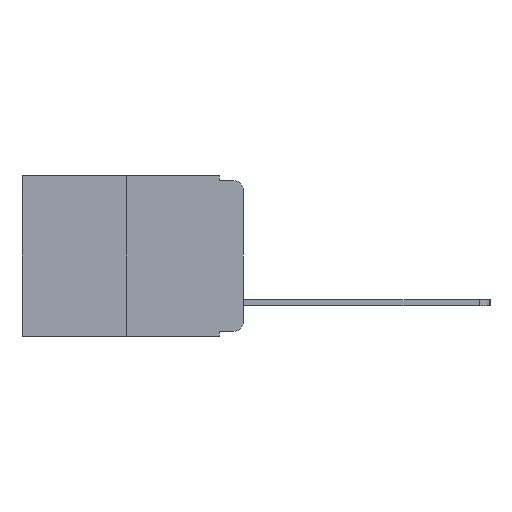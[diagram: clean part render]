
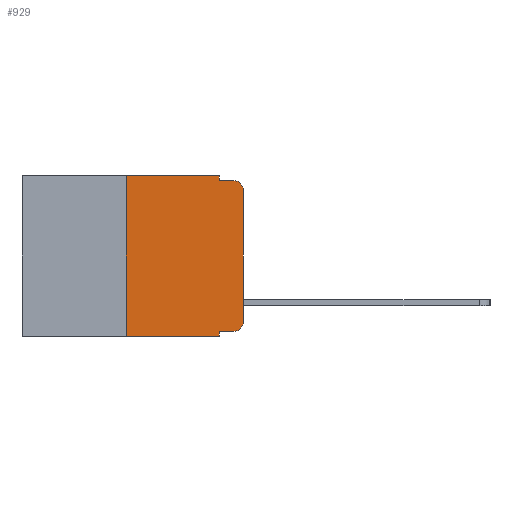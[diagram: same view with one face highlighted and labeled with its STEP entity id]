
A CAD part, left-side view. The second image highlights one B-rep face of the part: STEP entity #929.
In plain terms, the highlighted planar face has unit normal (-1, 0, 0).
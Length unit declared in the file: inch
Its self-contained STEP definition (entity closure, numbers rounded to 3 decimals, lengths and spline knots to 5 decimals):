
#144 = CARTESIAN_POINT ( 'NONE',  ( 0., 0.051, 0. ) ) ;
#150 = VECTOR ( 'NONE', #14400, 39.37008 ) ;
#474 = EDGE_CURVE ( 'NONE', #17470, #11154, #4488, .T. ) ;
#929 = ADVANCED_FACE ( 'NONE', ( #9199 ), #10557, .F. ) ;
#1122 = VERTEX_POINT ( 'NONE', #2299 ) ;
#1246 = CIRCLE ( 'NONE', #18736, 0.02 ) ;
#1361 = DIRECTION ( 'NONE',  ( -1., 0., 0. ) ) ;
#1369 = DIRECTION ( 'NONE',  ( 0., -1., 0. ) ) ;
#1697 = CARTESIAN_POINT ( 'NONE',  ( 0., 0.02, -0.03 ) ) ;
#2299 = CARTESIAN_POINT ( 'NONE',  ( 0., 0.051, -0.333 ) ) ;
#2404 = LINE ( 'NONE', #7173, #10400 ) ;
#2425 = DIRECTION ( 'NONE',  ( 0., 0., -1. ) ) ;
#2834 = VECTOR ( 'NONE', #5025, 39.37008 ) ;
#2888 = ORIENTED_EDGE ( 'NONE', *, *, #14302, .F. ) ;
#3519 = VECTOR ( 'NONE', #6937, 39.37008 ) ;
#3643 = ORIENTED_EDGE ( 'NONE', *, *, #13514, .F. ) ;
#4281 = CARTESIAN_POINT ( 'NONE',  ( 0., 0., -0.03 ) ) ;
#4284 = EDGE_CURVE ( 'NONE', #15797, #14308, #1246, .T. ) ;
#4296 = VERTEX_POINT ( 'NONE', #4281 ) ;
#4488 = LINE ( 'NONE', #10200, #150 ) ;
#4564 = CARTESIAN_POINT ( 'NONE',  ( 0., 0.051, -0.01 ) ) ;
#4687 = EDGE_CURVE ( 'NONE', #14308, #4296, #18473, .T. ) ;
#5025 = DIRECTION ( 'NONE',  ( 0., 0., -1. ) ) ;
#5111 = CARTESIAN_POINT ( 'NONE',  ( 0., 0.051, -0.01 ) ) ;
#5259 = VECTOR ( 'NONE', #11512, 39.37008 ) ;
#6584 = CARTESIAN_POINT ( 'NONE',  ( 0., 0.02, -0.01 ) ) ;
#6937 = DIRECTION ( 'NONE',  ( 0., -1., 0. ) ) ;
#6961 = ORIENTED_EDGE ( 'NONE', *, *, #14271, .F. ) ;
#7173 = CARTESIAN_POINT ( 'NONE',  ( 0., 0.473, 0. ) ) ;
#7245 = CARTESIAN_POINT ( 'NONE',  ( 0., 0.051, 0. ) ) ;
#7274 = EDGE_CURVE ( 'NONE', #4296, #20104, #8757, .T. ) ;
#7701 = ORIENTED_EDGE ( 'NONE', *, *, #12070, .T. ) ;
#7988 = DIRECTION ( 'NONE',  ( 1., 0., 0. ) ) ;
#8320 = VERTEX_POINT ( 'NONE', #14396 ) ;
#8325 = LINE ( 'NONE', #14064, #20124 ) ;
#8428 = DIRECTION ( 'NONE',  ( 0., 0., -1. ) ) ;
#8757 = CIRCLE ( 'NONE', #14910, 0.02 ) ;
#8801 = DIRECTION ( 'NONE',  ( 0., 0., -1. ) ) ;
#8940 = ORIENTED_EDGE ( 'NONE', *, *, #4284, .T. ) ;
#9199 = FACE_OUTER_BOUND ( 'NONE', #19956, .T. ) ;
#10200 = CARTESIAN_POINT ( 'NONE',  ( 0., 0.25, 0. ) ) ;
#10314 = DIRECTION ( 'NONE',  ( 0., -1., 0. ) ) ;
#10388 = CARTESIAN_POINT ( 'NONE',  ( 0., 0., -0.313 ) ) ;
#10400 = VECTOR ( 'NONE', #10314, 39.37008 ) ;
#10557 = PLANE ( 'NONE',  #14190 ) ;
#10722 = VECTOR ( 'NONE', #11204, 39.37008 ) ;
#11154 = VERTEX_POINT ( 'NONE', #12994 ) ;
#11204 = DIRECTION ( 'NONE',  ( 0., 0., 1. ) ) ;
#11381 = DIRECTION ( 'NONE',  ( -1., 0., 0. ) ) ;
#11512 = DIRECTION ( 'NONE',  ( 0., -1., 0. ) ) ;
#12070 = EDGE_CURVE ( 'NONE', #1122, #15797, #8325, .T. ) ;
#12297 = CARTESIAN_POINT ( 'NONE',  ( 0., 0.25, -0.343 ) ) ;
#12813 = VERTEX_POINT ( 'NONE', #144 ) ;
#12943 = EDGE_CURVE ( 'NONE', #17470, #8320, #16559, .T. ) ;
#12994 = CARTESIAN_POINT ( 'NONE',  ( 0., 0.25, 0. ) ) ;
#13514 = EDGE_CURVE ( 'NONE', #16378, #20104, #13611, .T. ) ;
#13562 = VECTOR ( 'NONE', #2425, 39.37008 ) ;
#13611 = LINE ( 'NONE', #5111, #5259 ) ;
#13987 = ORIENTED_EDGE ( 'NONE', *, *, #7274, .T. ) ;
#14026 = ORIENTED_EDGE ( 'NONE', *, *, #12943, .T. ) ;
#14064 = CARTESIAN_POINT ( 'NONE',  ( 0., 0.051, -0.333 ) ) ;
#14190 = AXIS2_PLACEMENT_3D ( 'NONE', #19953, #7988, #8428 ) ;
#14271 = EDGE_CURVE ( 'NONE', #11154, #12813, #2404, .T. ) ;
#14279 = ORIENTED_EDGE ( 'NONE', *, *, #474, .F. ) ;
#14302 = EDGE_CURVE ( 'NONE', #1122, #8320, #17711, .T. ) ;
#14308 = VERTEX_POINT ( 'NONE', #10388 ) ;
#14396 = CARTESIAN_POINT ( 'NONE',  ( 0., 0.051, -0.343 ) ) ;
#14400 = DIRECTION ( 'NONE',  ( 0., 0., 1. ) ) ;
#14740 = CARTESIAN_POINT ( 'NONE',  ( 0., 0., 0. ) ) ;
#14910 = AXIS2_PLACEMENT_3D ( 'NONE', #1697, #1361, #18112 ) ;
#15797 = VERTEX_POINT ( 'NONE', #19101 ) ;
#15909 = LINE ( 'NONE', #17557, #2834 ) ;
#16274 = CARTESIAN_POINT ( 'NONE',  ( 0., 0.473, -0.343 ) ) ;
#16378 = VERTEX_POINT ( 'NONE', #4564 ) ;
#16559 = LINE ( 'NONE', #16274, #3519 ) ;
#16932 = ORIENTED_EDGE ( 'NONE', *, *, #17066, .F. ) ;
#17066 = EDGE_CURVE ( 'NONE', #12813, #16378, #15909, .T. ) ;
#17470 = VERTEX_POINT ( 'NONE', #12297 ) ;
#17557 = CARTESIAN_POINT ( 'NONE',  ( 0., 0.051, 0. ) ) ;
#17711 = LINE ( 'NONE', #7245, #13562 ) ;
#17980 = CARTESIAN_POINT ( 'NONE',  ( 0., 0.02, -0.313 ) ) ;
#18112 = DIRECTION ( 'NONE',  ( 0., 0., -1. ) ) ;
#18137 = ORIENTED_EDGE ( 'NONE', *, *, #4687, .T. ) ;
#18473 = LINE ( 'NONE', #14740, #10722 ) ;
#18736 = AXIS2_PLACEMENT_3D ( 'NONE', #17980, #11381, #8801 ) ;
#19101 = CARTESIAN_POINT ( 'NONE',  ( 0., 0.02, -0.333 ) ) ;
#19953 = CARTESIAN_POINT ( 'NONE',  ( 0., 0.473, 0. ) ) ;
#19956 = EDGE_LOOP ( 'NONE', ( #18137, #13987, #3643, #16932, #6961, #14279, #14026, #2888, #7701, #8940 ) ) ;
#20104 = VERTEX_POINT ( 'NONE', #6584 ) ;
#20124 = VECTOR ( 'NONE', #1369, 39.37008 ) ;
